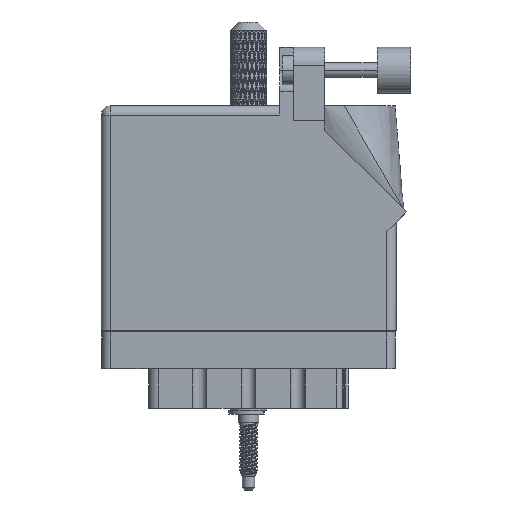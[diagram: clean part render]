
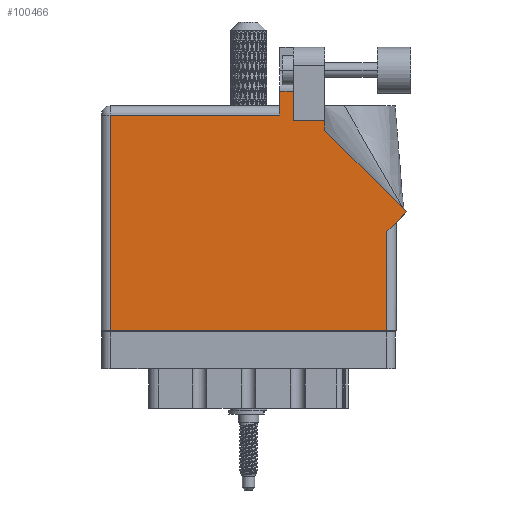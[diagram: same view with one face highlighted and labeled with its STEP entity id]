
A CAD part, front view. The second image highlights one B-rep face of the part: STEP entity #100466.
In plain terms, the highlighted face is planar.
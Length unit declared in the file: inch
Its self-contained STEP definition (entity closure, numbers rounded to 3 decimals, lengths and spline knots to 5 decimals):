
#1088 = CARTESIAN_POINT ( 'NONE',  ( 1.948, 0., 0. ) ) ;
#4577 = PLANE ( 'NONE',  #94919 ) ;
#4690 = VERTEX_POINT ( 'NONE', #60489 ) ;
#5051 = CARTESIAN_POINT ( 'NONE',  ( 0.062, 0., 0. ) ) ;
#5570 = EDGE_CURVE ( 'NONE', #58432, #49937, #93011, .T. ) ;
#5855 = VECTOR ( 'NONE', #103603, 39.37008 ) ;
#7824 = VERTEX_POINT ( 'NONE', #56823 ) ;
#8065 = CARTESIAN_POINT ( 'NONE',  ( 1.311, 1.43, 0. ) ) ;
#8106 = CARTESIAN_POINT ( 'NONE',  ( 1.524, 1.43, 0. ) ) ;
#10130 = VERTEX_POINT ( 'NONE', #22818 ) ;
#10200 = CARTESIAN_POINT ( 'NONE',  ( 2.08071, 0.80771, 0. ) ) ;
#18286 = ORIENTED_EDGE ( 'NONE', *, *, #72104, .T. ) ;
#18343 = ORIENTED_EDGE ( 'NONE', *, *, #65184, .T. ) ;
#20192 = CARTESIAN_POINT ( 'NONE',  ( 1.948, 0.737, 0. ) ) ;
#20346 = CARTESIAN_POINT ( 'NONE',  ( 1.311, 1.43, 0. ) ) ;
#20365 = CARTESIAN_POINT ( 'NONE',  ( 1.524, 1.43, 0. ) ) ;
#20906 = CARTESIAN_POINT ( 'NONE',  ( 0., 1.468, 0. ) ) ;
#20937 = VECTOR ( 'NONE', #51476, 39.37008 ) ;
#22818 = CARTESIAN_POINT ( 'NONE',  ( 1.217, 1.6315, 0. ) ) ;
#26917 = VECTOR ( 'NONE', #71302, 39.37008 ) ;
#28161 = VECTOR ( 'NONE', #78882, 39.37008 ) ;
#28558 = CARTESIAN_POINT ( 'NONE',  ( 0.062, 1.468, 0. ) ) ;
#29507 = LINE ( 'NONE', #5051, #26917 ) ;
#29624 = CARTESIAN_POINT ( 'NONE',  ( 1.217, 1.468, 0. ) ) ;
#30235 = LINE ( 'NONE', #10200, #61299 ) ;
#30901 = VECTOR ( 'NONE', #105781, 39.37008 ) ;
#32144 = LINE ( 'NONE', #65691, #65813 ) ;
#35451 = LINE ( 'NONE', #20192, #69173 ) ;
#36401 = VERTEX_POINT ( 'NONE', #80995 ) ;
#36725 = ORIENTED_EDGE ( 'NONE', *, *, #90102, .T. ) ;
#40380 = VERTEX_POINT ( 'NONE', #8065 ) ;
#40565 = CARTESIAN_POINT ( 'NONE',  ( 1.64177, 1.6315, 0. ) ) ;
#41400 = CARTESIAN_POINT ( 'NONE',  ( 1.524, 1.36442, 0. ) ) ;
#41490 = EDGE_CURVE ( 'NONE', #10130, #58432, #68244, .T. ) ;
#42958 = LINE ( 'NONE', #85162, #20937 ) ;
#46413 = EDGE_CURVE ( 'NONE', #85745, #91875, #42958, .T. ) ;
#46527 = DIRECTION ( 'NONE',  ( 0., 0., -1. ) ) ;
#49937 = VERTEX_POINT ( 'NONE', #28558 ) ;
#51476 = DIRECTION ( 'NONE',  ( 0., 1., 0. ) ) ;
#52755 = LINE ( 'NONE', #40565, #30901 ) ;
#53062 = ORIENTED_EDGE ( 'NONE', *, *, #104636, .T. ) ;
#53841 = EDGE_CURVE ( 'NONE', #36401, #85745, #30235, .T. ) ;
#55150 = ORIENTED_EDGE ( 'NONE', *, *, #41490, .T. ) ;
#55508 = DIRECTION ( 'NONE',  ( 0., -1., 0. ) ) ;
#56823 = CARTESIAN_POINT ( 'NONE',  ( 1.311, 1.6315, 0. ) ) ;
#58432 = VERTEX_POINT ( 'NONE', #29624 ) ;
#60489 = CARTESIAN_POINT ( 'NONE',  ( 1.948, 0.675, 0. ) ) ;
#61299 = VECTOR ( 'NONE', #95654, 39.37008 ) ;
#61325 = ORIENTED_EDGE ( 'NONE', *, *, #5570, .T. ) ;
#62453 = CARTESIAN_POINT ( 'NONE',  ( 0., 1.53, 0. ) ) ;
#63924 = LINE ( 'NONE', #20365, #105356 ) ;
#64174 = ORIENTED_EDGE ( 'NONE', *, *, #53841, .T. ) ;
#64928 = ORIENTED_EDGE ( 'NONE', *, *, #72368, .T. ) ;
#65184 = EDGE_CURVE ( 'NONE', #40380, #7824, #104191, .T. ) ;
#65691 = CARTESIAN_POINT ( 'NONE',  ( 0., 0., 0. ) ) ;
#65813 = VECTOR ( 'NONE', #83022, 39.37008 ) ;
#68244 = LINE ( 'NONE', #87738, #99268 ) ;
#68265 = VERTEX_POINT ( 'NONE', #81364 ) ;
#69173 = VECTOR ( 'NONE', #87903, 39.37008 ) ;
#71302 = DIRECTION ( 'NONE',  ( 0., -1., 0. ) ) ;
#72104 = EDGE_CURVE ( 'NONE', #7824, #10130, #52755, .T. ) ;
#72368 = EDGE_CURVE ( 'NONE', #49937, #68265, #29507, .T. ) ;
#78346 = DIRECTION ( 'NONE',  ( -1., 0., 0. ) ) ;
#78799 = DIRECTION ( 'NONE',  ( -1., 0., 0. ) ) ;
#78882 = DIRECTION ( 'NONE',  ( -1., 0., 0. ) ) ;
#80995 = CARTESIAN_POINT ( 'NONE',  ( 2.08071, 0.80771, 0. ) ) ;
#81364 = CARTESIAN_POINT ( 'NONE',  ( 0.062, 0., 0. ) ) ;
#83022 = DIRECTION ( 'NONE',  ( 1., 0., 0. ) ) ;
#83064 = ORIENTED_EDGE ( 'NONE', *, *, #99666, .T. ) ;
#83549 = EDGE_CURVE ( 'NONE', #4690, #36401, #83623, .T. ) ;
#83623 = LINE ( 'NONE', #84032, #91449 ) ;
#84032 = CARTESIAN_POINT ( 'NONE',  ( 2.01, 0.737, 0. ) ) ;
#85162 = CARTESIAN_POINT ( 'NONE',  ( 1.524, 1.36442, 0. ) ) ;
#85745 = VERTEX_POINT ( 'NONE', #41400 ) ;
#87194 = ORIENTED_EDGE ( 'NONE', *, *, #83549, .T. ) ;
#87738 = CARTESIAN_POINT ( 'NONE',  ( 1.217, 1.53, 0. ) ) ;
#87903 = DIRECTION ( 'NONE',  ( 0., 1., 0. ) ) ;
#90102 = EDGE_CURVE ( 'NONE', #96197, #4690, #35451, .T. ) ;
#91449 = VECTOR ( 'NONE', #100644, 39.37008 ) ;
#91875 = VERTEX_POINT ( 'NONE', #8106 ) ;
#93011 = LINE ( 'NONE', #20906, #28161 ) ;
#94919 = AXIS2_PLACEMENT_3D ( 'NONE', #62453, #46527, #78799 ) ;
#95654 = DIRECTION ( 'NONE',  ( -0.707, 0.707, 0. ) ) ;
#96135 = FACE_OUTER_BOUND ( 'NONE', #98156, .T. ) ;
#96197 = VERTEX_POINT ( 'NONE', #1088 ) ;
#98156 = EDGE_LOOP ( 'NONE', ( #18343, #18286, #55150, #61325, #64928, #53062, #36725, #87194, #64174, #106948, #83064 ) ) ;
#99268 = VECTOR ( 'NONE', #55508, 39.37008 ) ;
#99666 = EDGE_CURVE ( 'NONE', #91875, #40380, #63924, .T. ) ;
#100466 = ADVANCED_FACE ( 'NONE', ( #96135 ), #4577, .F. ) ;
#100644 = DIRECTION ( 'NONE',  ( 0.707, 0.707, 0. ) ) ;
#103603 = DIRECTION ( 'NONE',  ( 0., 1., 0. ) ) ;
#104191 = LINE ( 'NONE', #20346, #5855 ) ;
#104636 = EDGE_CURVE ( 'NONE', #68265, #96197, #32144, .T. ) ;
#105356 = VECTOR ( 'NONE', #78346, 39.37008 ) ;
#105781 = DIRECTION ( 'NONE',  ( -1., 0., 0. ) ) ;
#106948 = ORIENTED_EDGE ( 'NONE', *, *, #46413, .T. ) ;
